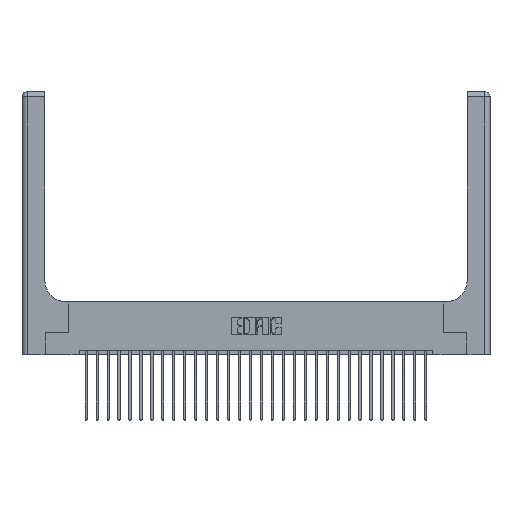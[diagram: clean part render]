
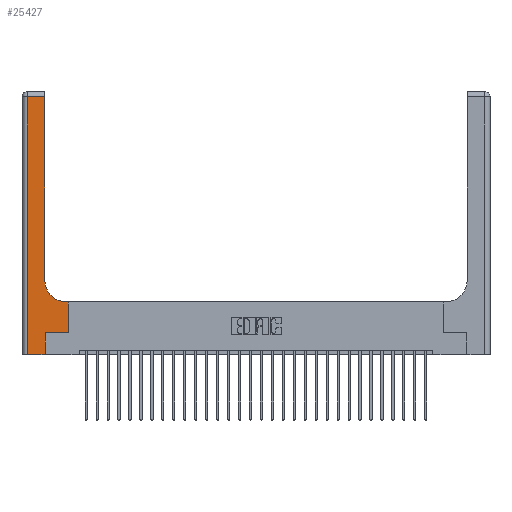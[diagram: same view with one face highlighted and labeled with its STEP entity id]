
A CAD part, top view. The second image highlights one B-rep face of the part: STEP entity #25427.
In plain terms, the highlighted planar face has unit normal (0, 0, 1).
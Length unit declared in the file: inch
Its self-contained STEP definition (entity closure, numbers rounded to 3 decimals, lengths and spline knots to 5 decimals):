
#475 = DIRECTION ( 'NONE',  ( 0., 0., -1. ) ) ;
#693 = ORIENTED_EDGE ( 'NONE', *, *, #21959, .T. ) ;
#1361 = LINE ( 'NONE', #15570, #13981 ) ;
#1388 = CARTESIAN_POINT ( 'NONE',  ( 0.528, 0.6, 0.37 ) ) ;
#1743 = VECTOR ( 'NONE', #5058, 39.37008 ) ;
#2139 = VERTEX_POINT ( 'NONE', #15142 ) ;
#2177 = DIRECTION ( 'NONE',  ( 0., 1., 0. ) ) ;
#2835 = EDGE_CURVE ( 'NONE', #6804, #19153, #1361, .T. ) ;
#3577 = DIRECTION ( 'NONE',  ( 0., 0., -1. ) ) ;
#4472 = LINE ( 'NONE', #24157, #19734 ) ;
#4517 = EDGE_CURVE ( 'NONE', #27374, #2139, #10861, .T. ) ;
#4748 = PLANE ( 'NONE',  #4960 ) ;
#4960 = AXIS2_PLACEMENT_3D ( 'NONE', #19375, #475, #17348 ) ;
#5058 = DIRECTION ( 'NONE',  ( 0., -1., 0. ) ) ;
#5167 = ORIENTED_EDGE ( 'NONE', *, *, #5942, .T. ) ;
#5501 = ORIENTED_EDGE ( 'NONE', *, *, #16333, .T. ) ;
#5716 = DIRECTION ( 'NONE',  ( 1., 0., 0. ) ) ;
#5942 = EDGE_CURVE ( 'NONE', #19153, #19312, #22589, .T. ) ;
#5977 = CARTESIAN_POINT ( 'NONE',  ( 0.51, 0.85, 0.37 ) ) ;
#6804 = VERTEX_POINT ( 'NONE', #9864 ) ;
#7120 = CARTESIAN_POINT ( 'NONE',  ( 0.265, 0., 0.37 ) ) ;
#7137 = LINE ( 'NONE', #20591, #11112 ) ;
#7491 = AXIS2_PLACEMENT_3D ( 'NONE', #5977, #3577, #5716 ) ;
#7512 = DIRECTION ( 'NONE',  ( -1., 0., 0. ) ) ;
#7708 = CARTESIAN_POINT ( 'NONE',  ( 0.26, 0.6, 0.37 ) ) ;
#9561 = CARTESIAN_POINT ( 'NONE',  ( 0.06, 2.94, 0.37 ) ) ;
#9836 = EDGE_LOOP ( 'NONE', ( #693, #25706, #12184, #5501, #21531, #26670, #5167, #26445, #22725 ) ) ;
#9864 = CARTESIAN_POINT ( 'NONE',  ( 0.265, 0.25, 0.37 ) ) ;
#10861 = CIRCLE ( 'NONE', #7491, 0.25 ) ;
#11100 = EDGE_CURVE ( 'NONE', #26740, #6804, #21312, .T. ) ;
#11112 = VECTOR ( 'NONE', #22807, 39.37008 ) ;
#11121 = DIRECTION ( 'NONE',  ( 1., 0., 0. ) ) ;
#12184 = ORIENTED_EDGE ( 'NONE', *, *, #24898, .T. ) ;
#12649 = VERTEX_POINT ( 'NONE', #24062 ) ;
#13981 = VECTOR ( 'NONE', #11121, 39.37008 ) ;
#14173 = CARTESIAN_POINT ( 'NONE',  ( 0.51, 0.6, 0.37 ) ) ;
#14198 = VERTEX_POINT ( 'NONE', #18438 ) ;
#14289 = VECTOR ( 'NONE', #2177, 39.37008 ) ;
#14642 = FACE_OUTER_BOUND ( 'NONE', #9836, .T. ) ;
#15142 = CARTESIAN_POINT ( 'NONE',  ( 0.26, 0.85, 0.37 ) ) ;
#15570 = CARTESIAN_POINT ( 'NONE',  ( 0.265, 0.25, 0.37 ) ) ;
#16333 = EDGE_CURVE ( 'NONE', #12649, #26740, #4472, .T. ) ;
#16517 = CARTESIAN_POINT ( 'NONE',  ( 0.265, 0., 0.37 ) ) ;
#16692 = EDGE_CURVE ( 'NONE', #14198, #20416, #7137, .T. ) ;
#17348 = DIRECTION ( 'NONE',  ( -1., 0., 0. ) ) ;
#18438 = CARTESIAN_POINT ( 'NONE',  ( 0.26, 2.94, 0.37 ) ) ;
#18883 = DIRECTION ( 'NONE',  ( 0., 1., 0. ) ) ;
#19098 = CARTESIAN_POINT ( 'NONE',  ( 0.528, 0.25, 0.37 ) ) ;
#19153 = VERTEX_POINT ( 'NONE', #19908 ) ;
#19312 = VERTEX_POINT ( 'NONE', #1388 ) ;
#19375 = CARTESIAN_POINT ( 'NONE',  ( 0., 3., 0.37 ) ) ;
#19703 = DIRECTION ( 'NONE',  ( 1., 0., 0. ) ) ;
#19734 = VECTOR ( 'NONE', #19703, 39.37008 ) ;
#19908 = CARTESIAN_POINT ( 'NONE',  ( 0.528, 0.25, 0.37 ) ) ;
#20062 = LINE ( 'NONE', #21188, #25686 ) ;
#20416 = VERTEX_POINT ( 'NONE', #9561 ) ;
#20591 = CARTESIAN_POINT ( 'NONE',  ( 0., 2.94, 0.37 ) ) ;
#20970 = LINE ( 'NONE', #7708, #24615 ) ;
#21188 = CARTESIAN_POINT ( 'NONE',  ( 0.26, 3., 0.37 ) ) ;
#21312 = LINE ( 'NONE', #16517, #26304 ) ;
#21531 = ORIENTED_EDGE ( 'NONE', *, *, #11100, .T. ) ;
#21959 = EDGE_CURVE ( 'NONE', #2139, #14198, #20062, .T. ) ;
#22589 = LINE ( 'NONE', #19098, #14289 ) ;
#22725 = ORIENTED_EDGE ( 'NONE', *, *, #4517, .T. ) ;
#22807 = DIRECTION ( 'NONE',  ( -1., 0., 0. ) ) ;
#24036 = CARTESIAN_POINT ( 'NONE',  ( 0.06, 3., 0.37 ) ) ;
#24043 = EDGE_CURVE ( 'NONE', #19312, #27374, #20970, .T. ) ;
#24062 = CARTESIAN_POINT ( 'NONE',  ( 0.06, 0., 0.37 ) ) ;
#24157 = CARTESIAN_POINT ( 'NONE',  ( 0., 0., 0.37 ) ) ;
#24280 = LINE ( 'NONE', #24036, #1743 ) ;
#24615 = VECTOR ( 'NONE', #7512, 39.37008 ) ;
#24744 = DIRECTION ( 'NONE',  ( 0., 1., 0. ) ) ;
#24898 = EDGE_CURVE ( 'NONE', #20416, #12649, #24280, .T. ) ;
#25427 = ADVANCED_FACE ( 'NONE', ( #14642 ), #4748, .F. ) ;
#25686 = VECTOR ( 'NONE', #18883, 39.37008 ) ;
#25706 = ORIENTED_EDGE ( 'NONE', *, *, #16692, .T. ) ;
#26304 = VECTOR ( 'NONE', #24744, 39.37008 ) ;
#26445 = ORIENTED_EDGE ( 'NONE', *, *, #24043, .T. ) ;
#26670 = ORIENTED_EDGE ( 'NONE', *, *, #2835, .T. ) ;
#26740 = VERTEX_POINT ( 'NONE', #7120 ) ;
#27374 = VERTEX_POINT ( 'NONE', #14173 ) ;
